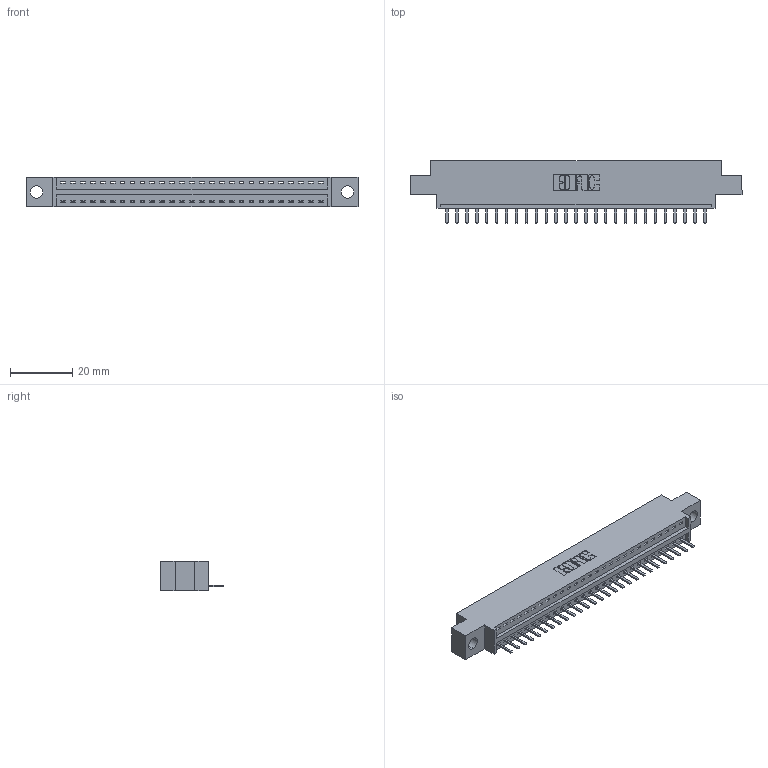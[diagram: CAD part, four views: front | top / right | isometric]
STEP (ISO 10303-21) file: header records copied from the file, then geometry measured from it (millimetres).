
FILE_DESCRIPTION (( 'STEP AP203' ), '1' );
FILE_NAME ('346-027-520-604.STEP', '2022-05-06T04:07:51', ( '' ), ( '' ), 'SwSTEP 2.0', 'SolidWorks 2020', '' );
FILE_SCHEMA (( 'CONFIG_CONTROL_DESIGN' ));
Length unit declared in the file: inch
Products named in the file (3): 345-292-001_345-293-120; 346-027-520-604; 346 Part_0.170 Offset - 0.156 Dia-TH
Assembly tree (28 placements, depth 2):
  346-027-520-604
    346 Part_0.170 Offset - 0.156 Dia-TH
    345-292-001_345-293-120  x27
Bounding box: 106.3 x 20.02 x 9.4 mm (x, y, z)
Volume: 9733.6 mm3; surface area: 11742.2 mm2
Topology: 28 solids, 28 shells, 1814 faces, 5345 edges, 3490 vertices
Faces by surface type: plane 1228, cylinder 586
Entity records: 19441 total; most frequent: CARTESIAN_POINT 3359, ORIENTED_EDGE 3306, DIRECTION 2967, EDGE_CURVE 1653, LINE 1409, VECTOR 1409, VERTEX_POINT 1098, AXIS2_PLACEMENT_3D 779
